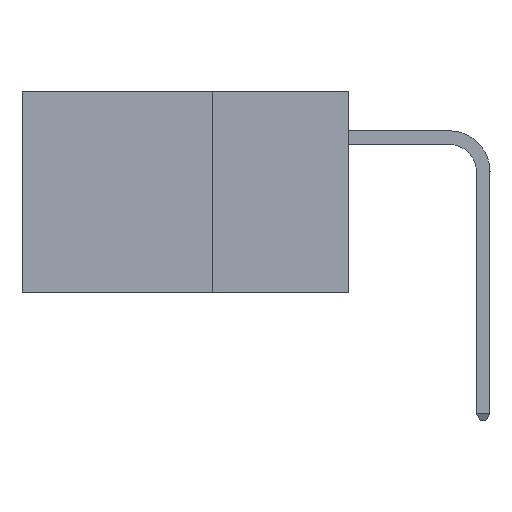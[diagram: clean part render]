
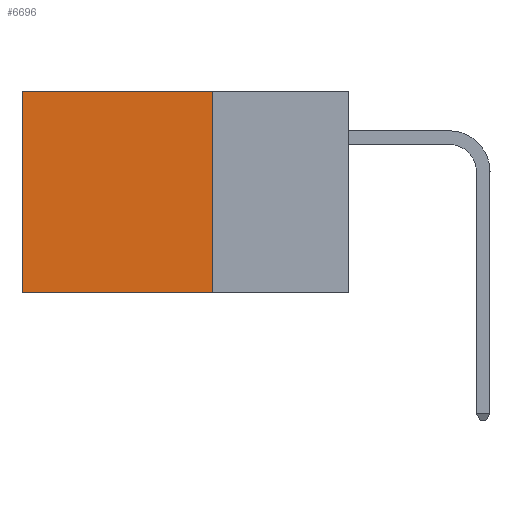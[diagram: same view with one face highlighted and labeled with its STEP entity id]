
A CAD part, left-side view. The second image highlights one B-rep face of the part: STEP entity #6696.
In plain terms, the highlighted planar face has unit normal (-1, 0, 0).
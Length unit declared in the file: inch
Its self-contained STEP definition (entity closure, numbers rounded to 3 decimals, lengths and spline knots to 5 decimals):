
#852 = CARTESIAN_POINT ( 'NONE',  ( 0.2875, 0.6, 0. ) ) ;
#1141 = CARTESIAN_POINT ( 'NONE',  ( 0.2875, 0.25, 0. ) ) ;
#1315 = VECTOR ( 'NONE', #14986, 39.37008 ) ;
#1362 = VECTOR ( 'NONE', #21118, 39.37008 ) ;
#1949 = ORIENTED_EDGE ( 'NONE', *, *, #13647, .F. ) ;
#2234 = DIRECTION ( 'NONE',  ( 0., 1., 0. ) ) ;
#4452 = CARTESIAN_POINT ( 'NONE',  ( 0.2875, 0.6, -0.37 ) ) ;
#4777 = CARTESIAN_POINT ( 'NONE',  ( 0.2875, 0.25, -0.37 ) ) ;
#5060 = LINE ( 'NONE', #852, #1315 ) ;
#5596 = VERTEX_POINT ( 'NONE', #1141 ) ;
#5841 = FACE_OUTER_BOUND ( 'NONE', #9008, .T. ) ;
#6644 = CARTESIAN_POINT ( 'NONE',  ( 0.2875, 0.25, 0. ) ) ;
#6696 = ADVANCED_FACE ( 'NONE', ( #5841 ), #8440, .F. ) ;
#6737 = VERTEX_POINT ( 'NONE', #4777 ) ;
#7245 = LINE ( 'NONE', #19860, #20186 ) ;
#8333 = ORIENTED_EDGE ( 'NONE', *, *, #14681, .F. ) ;
#8412 = DIRECTION ( 'NONE',  ( 1., 0., 0. ) ) ;
#8440 = PLANE ( 'NONE',  #21395 ) ;
#8473 = ORIENTED_EDGE ( 'NONE', *, *, #11415, .T. ) ;
#8627 = DIRECTION ( 'NONE',  ( 0., 0., -1. ) ) ;
#9008 = EDGE_LOOP ( 'NONE', ( #8473, #8333, #1949, #20614 ) ) ;
#9412 = CARTESIAN_POINT ( 'NONE',  ( 0.2875, 0.25, 0. ) ) ;
#11415 = EDGE_CURVE ( 'NONE', #15167, #15437, #5060, .T. ) ;
#12106 = LINE ( 'NONE', #16199, #15986 ) ;
#13647 = EDGE_CURVE ( 'NONE', #5596, #6737, #7245, .T. ) ;
#14681 = EDGE_CURVE ( 'NONE', #6737, #15437, #12106, .T. ) ;
#14871 = LINE ( 'NONE', #9412, #1362 ) ;
#14951 = DIRECTION ( 'NONE',  ( 0., 0., -1. ) ) ;
#14986 = DIRECTION ( 'NONE',  ( 0., 0., -1. ) ) ;
#15167 = VERTEX_POINT ( 'NONE', #22403 ) ;
#15437 = VERTEX_POINT ( 'NONE', #4452 ) ;
#15986 = VECTOR ( 'NONE', #2234, 39.37008 ) ;
#16199 = CARTESIAN_POINT ( 'NONE',  ( 0.2875, 0.25, -0.37 ) ) ;
#19860 = CARTESIAN_POINT ( 'NONE',  ( 0.2875, 0.25, 0. ) ) ;
#20186 = VECTOR ( 'NONE', #14951, 39.37008 ) ;
#20614 = ORIENTED_EDGE ( 'NONE', *, *, #21578, .T. ) ;
#21118 = DIRECTION ( 'NONE',  ( 0., 1., 0. ) ) ;
#21395 = AXIS2_PLACEMENT_3D ( 'NONE', #6644, #8412, #8627 ) ;
#21578 = EDGE_CURVE ( 'NONE', #5596, #15167, #14871, .T. ) ;
#22403 = CARTESIAN_POINT ( 'NONE',  ( 0.2875, 0.6, 0. ) ) ;
